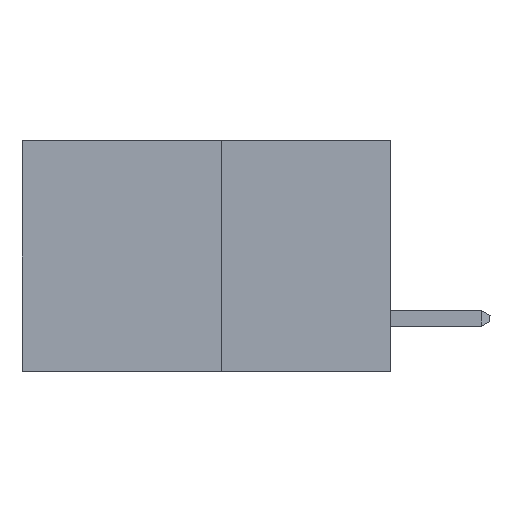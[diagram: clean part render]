
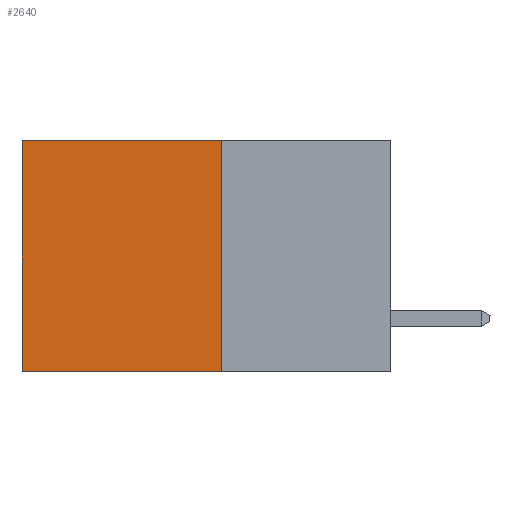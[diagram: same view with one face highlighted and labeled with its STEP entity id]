
A CAD part, left-side view. The second image highlights one B-rep face of the part: STEP entity #2640.
In plain terms, the highlighted planar face has unit normal (-1, 0, 0).
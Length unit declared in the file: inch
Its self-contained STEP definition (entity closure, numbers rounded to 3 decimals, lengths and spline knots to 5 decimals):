
#216 = EDGE_LOOP ( 'NONE', ( #2865, #3669, #349, #226 ) ) ;
#226 = ORIENTED_EDGE ( 'NONE', *, *, #8954, .T. ) ;
#349 = ORIENTED_EDGE ( 'NONE', *, *, #492, .F. ) ;
#357 = CARTESIAN_POINT ( 'NONE',  ( 0.277, 0.59, -0.37 ) ) ;
#459 = DIRECTION ( 'NONE',  ( 0., 0., -1. ) ) ;
#492 = EDGE_CURVE ( 'NONE', #5016, #3568, #4560, .T. ) ;
#540 = VERTEX_POINT ( 'NONE', #6678 ) ;
#1163 = CARTESIAN_POINT ( 'NONE',  ( 0.277, 0.27, 0. ) ) ;
#1391 = CARTESIAN_POINT ( 'NONE',  ( 0.277, 0.27, -0.37 ) ) ;
#1427 = EDGE_CURVE ( 'NONE', #3568, #5795, #6688, .T. ) ;
#2110 = DIRECTION ( 'NONE',  ( 0., 1., 0. ) ) ;
#2639 = LINE ( 'NONE', #357, #4589 ) ;
#2640 = ADVANCED_FACE ( 'NONE', ( #4481 ), #8931, .F. ) ;
#2865 = ORIENTED_EDGE ( 'NONE', *, *, #3753, .T. ) ;
#3460 = LINE ( 'NONE', #1163, #8778 ) ;
#3568 = VERTEX_POINT ( 'NONE', #1391 ) ;
#3669 = ORIENTED_EDGE ( 'NONE', *, *, #1427, .F. ) ;
#3753 = EDGE_CURVE ( 'NONE', #540, #5795, #2639, .T. ) ;
#4481 = FACE_OUTER_BOUND ( 'NONE', #216, .T. ) ;
#4560 = LINE ( 'NONE', #5338, #8052 ) ;
#4589 = VECTOR ( 'NONE', #459, 39.37008 ) ;
#4761 = VECTOR ( 'NONE', #8836, 39.37008 ) ;
#5016 = VERTEX_POINT ( 'NONE', #7985 ) ;
#5048 = CARTESIAN_POINT ( 'NONE',  ( 0.277, 0.27, -0.37 ) ) ;
#5338 = CARTESIAN_POINT ( 'NONE',  ( 0.277, 0.27, -0.37 ) ) ;
#5795 = VERTEX_POINT ( 'NONE', #7944 ) ;
#6678 = CARTESIAN_POINT ( 'NONE',  ( 0.277, 0.59, 0. ) ) ;
#6688 = LINE ( 'NONE', #5048, #4761 ) ;
#7944 = CARTESIAN_POINT ( 'NONE',  ( 0.277, 0.59, -0.37 ) ) ;
#7985 = CARTESIAN_POINT ( 'NONE',  ( 0.277, 0.27, 0. ) ) ;
#8052 = VECTOR ( 'NONE', #9481, 39.37008 ) ;
#8778 = VECTOR ( 'NONE', #2110, 39.37008 ) ;
#8836 = DIRECTION ( 'NONE',  ( 0., 1., 0. ) ) ;
#8881 = DIRECTION ( 'NONE',  ( 0., 0., -1. ) ) ;
#8883 = DIRECTION ( 'NONE',  ( 1., 0., 0. ) ) ;
#8931 = PLANE ( 'NONE',  #9434 ) ;
#8954 = EDGE_CURVE ( 'NONE', #5016, #540, #3460, .T. ) ;
#9063 = CARTESIAN_POINT ( 'NONE',  ( 0.277, 0.27, -0.37 ) ) ;
#9434 = AXIS2_PLACEMENT_3D ( 'NONE', #9063, #8883, #8881 ) ;
#9481 = DIRECTION ( 'NONE',  ( 0., 0., -1. ) ) ;
